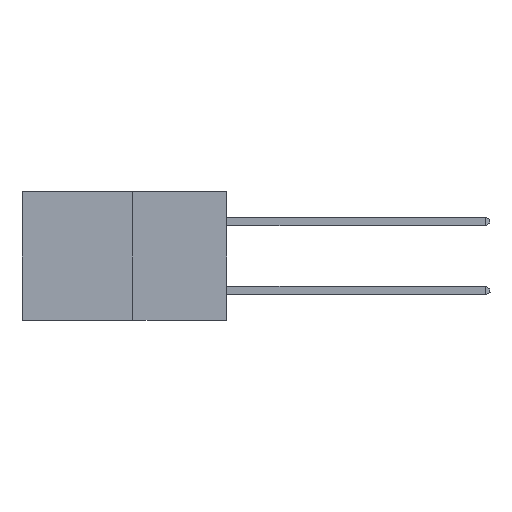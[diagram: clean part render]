
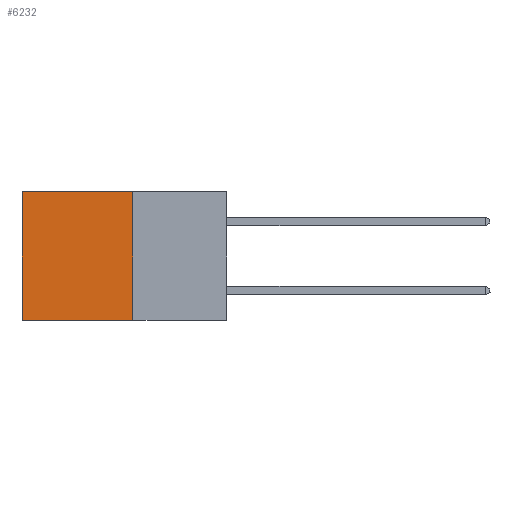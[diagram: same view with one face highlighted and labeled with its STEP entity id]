
A CAD part, left-side view. The second image highlights one B-rep face of the part: STEP entity #6232.
In plain terms, the highlighted planar face has unit normal (-1, 0, 0).
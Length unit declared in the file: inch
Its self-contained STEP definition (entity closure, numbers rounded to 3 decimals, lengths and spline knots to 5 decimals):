
#118 = VECTOR ( 'NONE', #7138, 39.37008 ) ;
#124 = PLANE ( 'NONE',  #3403 ) ;
#221 = DIRECTION ( 'NONE',  ( 0., 0., -1. ) ) ;
#622 = VECTOR ( 'NONE', #16282, 39.37008 ) ;
#1339 = VECTOR ( 'NONE', #22147, 39.37008 ) ;
#1387 = CARTESIAN_POINT ( 'NONE',  ( 0.277, 0.59, 0. ) ) ;
#1401 = CARTESIAN_POINT ( 'NONE',  ( 0.277, 0.27, 0. ) ) ;
#3307 = CARTESIAN_POINT ( 'NONE',  ( 0.277, 0.59, -0.37 ) ) ;
#3360 = CARTESIAN_POINT ( 'NONE',  ( 0.277, 0.59, -0.37 ) ) ;
#3403 = AXIS2_PLACEMENT_3D ( 'NONE', #22728, #11498, #221 ) ;
#3537 = CARTESIAN_POINT ( 'NONE',  ( 0.277, 0.27, -0.37 ) ) ;
#4616 = FACE_OUTER_BOUND ( 'NONE', #23004, .T. ) ;
#5042 = ORIENTED_EDGE ( 'NONE', *, *, #12323, .T. ) ;
#5260 = CARTESIAN_POINT ( 'NONE',  ( 0.277, 0.27, 0. ) ) ;
#5628 = LINE ( 'NONE', #23695, #622 ) ;
#6232 = ADVANCED_FACE ( 'NONE', ( #4616 ), #124, .F. ) ;
#6603 = CARTESIAN_POINT ( 'NONE',  ( 0.277, 0.27, -0.37 ) ) ;
#7138 = DIRECTION ( 'NONE',  ( 0., 1., 0. ) ) ;
#7774 = VERTEX_POINT ( 'NONE', #6603 ) ;
#7933 = VERTEX_POINT ( 'NONE', #1401 ) ;
#9171 = VECTOR ( 'NONE', #18587, 39.37008 ) ;
#11498 = DIRECTION ( 'NONE',  ( 1., 0., 0. ) ) ;
#12323 = EDGE_CURVE ( 'NONE', #7933, #19485, #15169, .T. ) ;
#13322 = ORIENTED_EDGE ( 'NONE', *, *, #23528, .F. ) ;
#14264 = ORIENTED_EDGE ( 'NONE', *, *, #20820, .T. ) ;
#15169 = LINE ( 'NONE', #5260, #118 ) ;
#16282 = DIRECTION ( 'NONE',  ( 0., 1., 0. ) ) ;
#16961 = LINE ( 'NONE', #3360, #1339 ) ;
#18587 = DIRECTION ( 'NONE',  ( 0., 0., -1. ) ) ;
#19485 = VERTEX_POINT ( 'NONE', #1387 ) ;
#20806 = ORIENTED_EDGE ( 'NONE', *, *, #22987, .F. ) ;
#20820 = EDGE_CURVE ( 'NONE', #19485, #22037, #16961, .T. ) ;
#22037 = VERTEX_POINT ( 'NONE', #3307 ) ;
#22147 = DIRECTION ( 'NONE',  ( 0., 0., -1. ) ) ;
#22728 = CARTESIAN_POINT ( 'NONE',  ( 0.277, 0.27, -0.37 ) ) ;
#22987 = EDGE_CURVE ( 'NONE', #7933, #7774, #23540, .T. ) ;
#23004 = EDGE_LOOP ( 'NONE', ( #14264, #13322, #20806, #5042 ) ) ;
#23528 = EDGE_CURVE ( 'NONE', #7774, #22037, #5628, .T. ) ;
#23540 = LINE ( 'NONE', #3537, #9171 ) ;
#23695 = CARTESIAN_POINT ( 'NONE',  ( 0.277, 0.27, -0.37 ) ) ;
